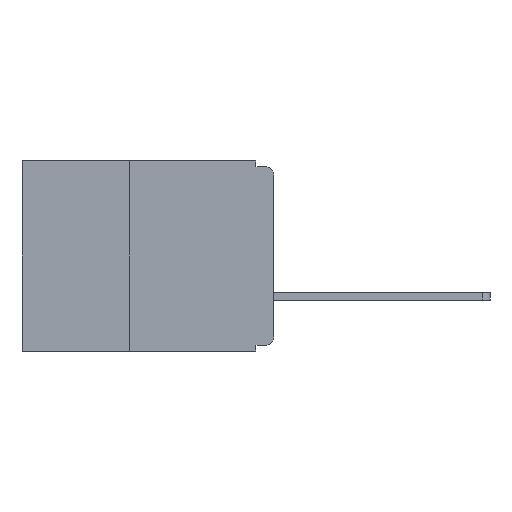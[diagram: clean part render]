
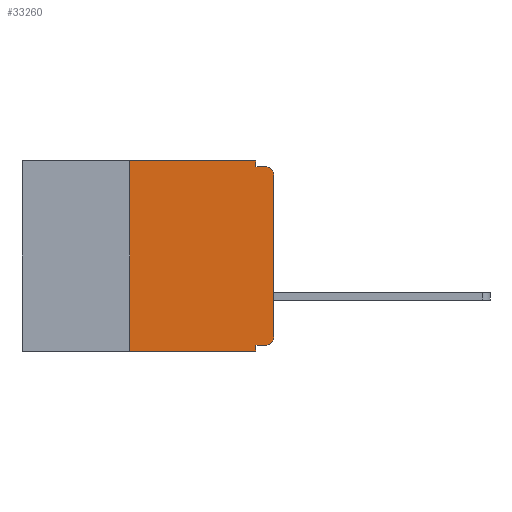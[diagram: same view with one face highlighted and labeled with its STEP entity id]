
A CAD part, left-side view. The second image highlights one B-rep face of the part: STEP entity #33260.
In plain terms, the highlighted planar face has unit normal (-1, 0, 0).
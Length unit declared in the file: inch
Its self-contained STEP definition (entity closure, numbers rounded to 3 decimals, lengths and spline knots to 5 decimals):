
#46 = AXIS2_PLACEMENT_3D ( 'NONE', #23305, #7792, #25925 ) ;
#275 = LINE ( 'NONE', #6533, #6564 ) ;
#355 = DIRECTION ( 'NONE',  ( -1., 0., 0. ) ) ;
#995 = DIRECTION ( 'NONE',  ( 0., 0., -1. ) ) ;
#1200 = VERTEX_POINT ( 'NONE', #32503 ) ;
#3042 = CARTESIAN_POINT ( 'NONE',  ( 0., 0., -0.025 ) ) ;
#3344 = VERTEX_POINT ( 'NONE', #33212 ) ;
#3621 = CARTESIAN_POINT ( 'NONE',  ( 0., 0.031, -0.32 ) ) ;
#3796 = EDGE_CURVE ( 'NONE', #26177, #18570, #275, .T. ) ;
#3979 = CARTESIAN_POINT ( 'NONE',  ( 0., 0.031, -0.01 ) ) ;
#4199 = ORIENTED_EDGE ( 'NONE', *, *, #24241, .T. ) ;
#4317 = CIRCLE ( 'NONE', #46, 0.015 ) ;
#5516 = DIRECTION ( 'NONE',  ( 0., 0., -1. ) ) ;
#5838 = VERTEX_POINT ( 'NONE', #20913 ) ;
#6533 = CARTESIAN_POINT ( 'NONE',  ( 0., 0.031, -0.33 ) ) ;
#6564 = VECTOR ( 'NONE', #5516, 39.37008 ) ;
#6817 = LINE ( 'NONE', #29305, #32867 ) ;
#6943 = ORIENTED_EDGE ( 'NONE', *, *, #10747, .F. ) ;
#7355 = VERTEX_POINT ( 'NONE', #19631 ) ;
#7792 = DIRECTION ( 'NONE',  ( -1., 0., 0. ) ) ;
#8191 = VECTOR ( 'NONE', #995, 39.37008 ) ;
#8479 = ORIENTED_EDGE ( 'NONE', *, *, #26772, .T. ) ;
#9091 = FACE_OUTER_BOUND ( 'NONE', #12361, .T. ) ;
#9427 = VERTEX_POINT ( 'NONE', #26280 ) ;
#10155 = VERTEX_POINT ( 'NONE', #3979 ) ;
#10252 = DIRECTION ( 'NONE',  ( 0., 0., -1. ) ) ;
#10491 = CARTESIAN_POINT ( 'NONE',  ( 0., 0.031, -0.33 ) ) ;
#10747 = EDGE_CURVE ( 'NONE', #13034, #10155, #21965, .T. ) ;
#11038 = ORIENTED_EDGE ( 'NONE', *, *, #22467, .F. ) ;
#12361 = EDGE_LOOP ( 'NONE', ( #8479, #21580, #11038, #6943, #22220, #32692, #4199, #32260, #25902, #26555 ) ) ;
#12760 = EDGE_CURVE ( 'NONE', #9427, #1200, #14248, .T. ) ;
#12982 = DIRECTION ( 'NONE',  ( 0., 0., 1. ) ) ;
#13034 = VERTEX_POINT ( 'NONE', #19867 ) ;
#13115 = LINE ( 'NONE', #13169, #26025 ) ;
#13169 = CARTESIAN_POINT ( 'NONE',  ( 0., 0., -0.01 ) ) ;
#13273 = AXIS2_PLACEMENT_3D ( 'NONE', #23145, #25769, #10252 ) ;
#13445 = LINE ( 'NONE', #14246, #26365 ) ;
#13971 = VECTOR ( 'NONE', #31342, 39.37008 ) ;
#14109 = CARTESIAN_POINT ( 'NONE',  ( 0., 0.031, 0. ) ) ;
#14246 = CARTESIAN_POINT ( 'NONE',  ( 0., 0., -0.32 ) ) ;
#14248 = CIRCLE ( 'NONE', #26917, 0.015 ) ;
#14941 = EDGE_CURVE ( 'NONE', #5838, #7355, #16462, .T. ) ;
#15764 = DIRECTION ( 'NONE',  ( 0., -1., 0. ) ) ;
#15808 = CARTESIAN_POINT ( 'NONE',  ( 0., 0., 0. ) ) ;
#15986 = EDGE_CURVE ( 'NONE', #7355, #13034, #21655, .T. ) ;
#16183 = CARTESIAN_POINT ( 'NONE',  ( 0., 0.015, -0.305 ) ) ;
#16462 = LINE ( 'NONE', #28499, #29442 ) ;
#16832 = DIRECTION ( 'NONE',  ( 0., 1., 0. ) ) ;
#18570 = VERTEX_POINT ( 'NONE', #10491 ) ;
#18778 = DIRECTION ( 'NONE',  ( 0., 0., -1. ) ) ;
#19631 = CARTESIAN_POINT ( 'NONE',  ( 0., 0.25, 0. ) ) ;
#19867 = CARTESIAN_POINT ( 'NONE',  ( 0., 0.031, 0. ) ) ;
#20432 = DIRECTION ( 'NONE',  ( 0., -1., 0. ) ) ;
#20834 = VECTOR ( 'NONE', #20432, 39.37008 ) ;
#20913 = CARTESIAN_POINT ( 'NONE',  ( 0., 0.25, -0.33 ) ) ;
#21541 = DIRECTION ( 'NONE',  ( 0., -1., 0. ) ) ;
#21580 = ORIENTED_EDGE ( 'NONE', *, *, #28726, .T. ) ;
#21655 = LINE ( 'NONE', #23000, #20834 ) ;
#21965 = LINE ( 'NONE', #14109, #8191 ) ;
#22220 = ORIENTED_EDGE ( 'NONE', *, *, #15986, .F. ) ;
#22467 = EDGE_CURVE ( 'NONE', #10155, #3344, #13115, .T. ) ;
#23000 = CARTESIAN_POINT ( 'NONE',  ( 0., 0.437, 0. ) ) ;
#23145 = CARTESIAN_POINT ( 'NONE',  ( 0., 0.437, 0. ) ) ;
#23305 = CARTESIAN_POINT ( 'NONE',  ( 0., 0.015, -0.025 ) ) ;
#24241 = EDGE_CURVE ( 'NONE', #5838, #18570, #6817, .T. ) ;
#25769 = DIRECTION ( 'NONE',  ( 1., 0., 0. ) ) ;
#25902 = ORIENTED_EDGE ( 'NONE', *, *, #28386, .F. ) ;
#25925 = DIRECTION ( 'NONE',  ( 0., 0., -1. ) ) ;
#26024 = VERTEX_POINT ( 'NONE', #3042 ) ;
#26025 = VECTOR ( 'NONE', #15764, 39.37008 ) ;
#26177 = VERTEX_POINT ( 'NONE', #3621 ) ;
#26280 = CARTESIAN_POINT ( 'NONE',  ( 0., 0.015, -0.32 ) ) ;
#26365 = VECTOR ( 'NONE', #16832, 39.37008 ) ;
#26555 = ORIENTED_EDGE ( 'NONE', *, *, #12760, .T. ) ;
#26772 = EDGE_CURVE ( 'NONE', #1200, #26024, #28539, .T. ) ;
#26917 = AXIS2_PLACEMENT_3D ( 'NONE', #16183, #355, #18778 ) ;
#28386 = EDGE_CURVE ( 'NONE', #9427, #26177, #13445, .T. ) ;
#28499 = CARTESIAN_POINT ( 'NONE',  ( 0., 0.25, -0.33 ) ) ;
#28539 = LINE ( 'NONE', #15808, #13971 ) ;
#28726 = EDGE_CURVE ( 'NONE', #26024, #3344, #4317, .T. ) ;
#29305 = CARTESIAN_POINT ( 'NONE',  ( 0., 0.437, -0.33 ) ) ;
#29442 = VECTOR ( 'NONE', #12982, 39.37008 ) ;
#31342 = DIRECTION ( 'NONE',  ( 0., 0., 1. ) ) ;
#32260 = ORIENTED_EDGE ( 'NONE', *, *, #3796, .F. ) ;
#32503 = CARTESIAN_POINT ( 'NONE',  ( 0., 0., -0.305 ) ) ;
#32692 = ORIENTED_EDGE ( 'NONE', *, *, #14941, .F. ) ;
#32867 = VECTOR ( 'NONE', #21541, 39.37008 ) ;
#33212 = CARTESIAN_POINT ( 'NONE',  ( 0., 0.015, -0.01 ) ) ;
#33260 = ADVANCED_FACE ( 'NONE', ( #9091 ), #33569, .F. ) ;
#33569 = PLANE ( 'NONE',  #13273 ) ;
